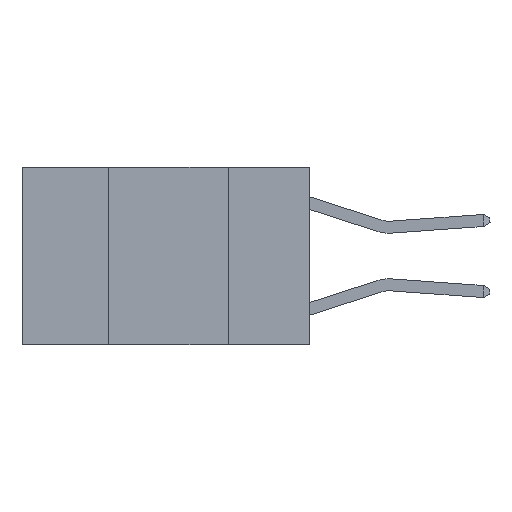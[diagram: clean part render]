
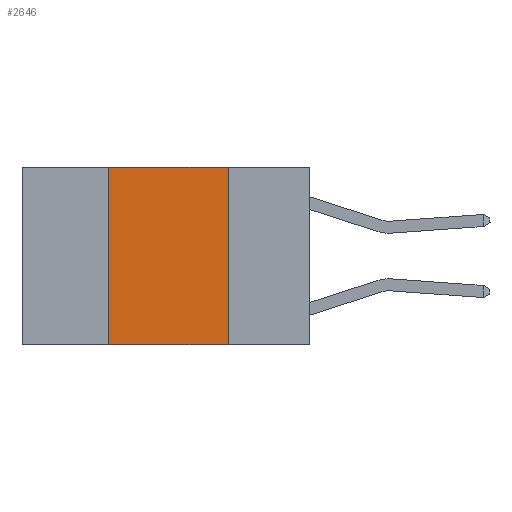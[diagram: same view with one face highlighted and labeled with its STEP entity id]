
A CAD part, left-side view. The second image highlights one B-rep face of the part: STEP entity #2646.
In plain terms, the highlighted planar face has unit normal (-1, 0, 0).
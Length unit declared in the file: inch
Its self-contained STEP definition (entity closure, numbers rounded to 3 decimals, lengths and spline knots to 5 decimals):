
#74 = CARTESIAN_POINT ( 'NONE',  ( 0., 0.6, -0.37 ) ) ;
#1054 = DIRECTION ( 'NONE',  ( 0., -1., 0. ) ) ;
#1122 = EDGE_CURVE ( 'NONE', #3375, #7797, #9461, .T. ) ;
#1296 = CARTESIAN_POINT ( 'NONE',  ( 0., 0.42, 0. ) ) ;
#1782 = ORIENTED_EDGE ( 'NONE', *, *, #6755, .F. ) ;
#2008 = CARTESIAN_POINT ( 'NONE',  ( 0., 0.17, 0. ) ) ;
#2201 = DIRECTION ( 'NONE',  ( 0., 0., 1. ) ) ;
#2291 = LINE ( 'NONE', #9252, #9050 ) ;
#2312 = EDGE_CURVE ( 'NONE', #3375, #5555, #3730, .T. ) ;
#2646 = ADVANCED_FACE ( 'NONE', ( #8589 ), #5224, .F. ) ;
#3375 = VERTEX_POINT ( 'NONE', #10893 ) ;
#3730 = LINE ( 'NONE', #74, #10611 ) ;
#3993 = EDGE_CURVE ( 'NONE', #4372, #5555, #6016, .T. ) ;
#4232 = DIRECTION ( 'NONE',  ( 0., -1., 0. ) ) ;
#4370 = CARTESIAN_POINT ( 'NONE',  ( 0., 0.6, 0. ) ) ;
#4372 = VERTEX_POINT ( 'NONE', #2008 ) ;
#4503 = EDGE_LOOP ( 'NONE', ( #6218, #1782, #9494, #6257 ) ) ;
#4996 = DIRECTION ( 'NONE',  ( 0., 0., -1. ) ) ;
#5224 = PLANE ( 'NONE',  #6490 ) ;
#5555 = VERTEX_POINT ( 'NONE', #11188 ) ;
#5778 = VECTOR ( 'NONE', #4996, 39.37008 ) ;
#6016 = LINE ( 'NONE', #7536, #5778 ) ;
#6218 = ORIENTED_EDGE ( 'NONE', *, *, #3993, .F. ) ;
#6257 = ORIENTED_EDGE ( 'NONE', *, *, #2312, .T. ) ;
#6490 = AXIS2_PLACEMENT_3D ( 'NONE', #4370, #7855, #7174 ) ;
#6755 = EDGE_CURVE ( 'NONE', #7797, #4372, #2291, .T. ) ;
#7174 = DIRECTION ( 'NONE',  ( 0., 0., -1. ) ) ;
#7394 = VECTOR ( 'NONE', #2201, 39.37008 ) ;
#7536 = CARTESIAN_POINT ( 'NONE',  ( 0., 0.17, 0. ) ) ;
#7797 = VERTEX_POINT ( 'NONE', #1296 ) ;
#7855 = DIRECTION ( 'NONE',  ( 1., 0., 0. ) ) ;
#8589 = FACE_OUTER_BOUND ( 'NONE', #4503, .T. ) ;
#9050 = VECTOR ( 'NONE', #4232, 39.37008 ) ;
#9252 = CARTESIAN_POINT ( 'NONE',  ( 0., 0.6, 0. ) ) ;
#9461 = LINE ( 'NONE', #9959, #7394 ) ;
#9494 = ORIENTED_EDGE ( 'NONE', *, *, #1122, .F. ) ;
#9959 = CARTESIAN_POINT ( 'NONE',  ( 0., 0.42, 0. ) ) ;
#10611 = VECTOR ( 'NONE', #1054, 39.37008 ) ;
#10893 = CARTESIAN_POINT ( 'NONE',  ( 0., 0.42, -0.37 ) ) ;
#11188 = CARTESIAN_POINT ( 'NONE',  ( 0., 0.17, -0.37 ) ) ;
